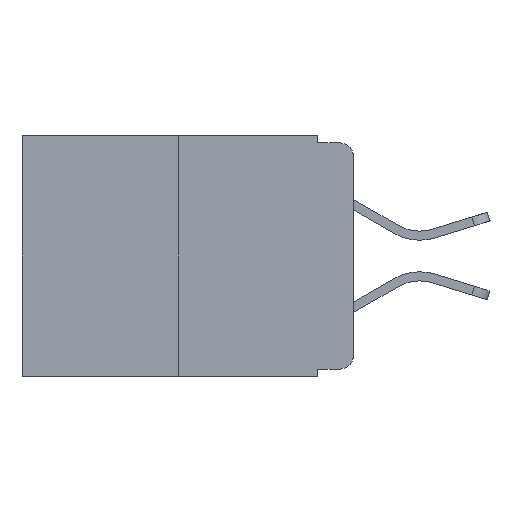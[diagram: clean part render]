
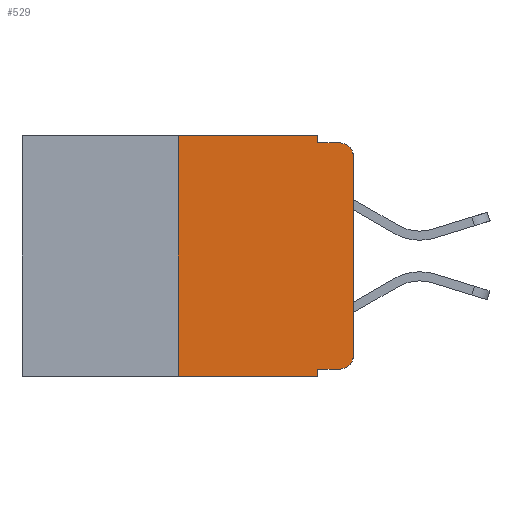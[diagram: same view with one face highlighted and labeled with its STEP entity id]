
A CAD part, left-side view. The second image highlights one B-rep face of the part: STEP entity #529.
In plain terms, the highlighted planar face has unit normal (-1, 0, 0).
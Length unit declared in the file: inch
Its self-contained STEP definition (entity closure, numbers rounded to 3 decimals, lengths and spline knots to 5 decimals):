
#18 = ORIENTED_EDGE ( 'NONE', *, *, #6493, .T. ) ;
#202 = DIRECTION ( 'NONE',  ( 0., 0., 1. ) ) ;
#225 = VERTEX_POINT ( 'NONE', #7910 ) ;
#264 = VERTEX_POINT ( 'NONE', #2748 ) ;
#381 = DIRECTION ( 'NONE',  ( 0., 0., -1. ) ) ;
#408 = VECTOR ( 'NONE', #202, 39.37008 ) ;
#529 = ADVANCED_FACE ( 'NONE', ( #13512 ), #13911, .F. ) ;
#679 = ORIENTED_EDGE ( 'NONE', *, *, #18257, .T. ) ;
#880 = EDGE_CURVE ( 'NONE', #6363, #5729, #3948, .T. ) ;
#1141 = DIRECTION ( 'NONE',  ( 0., 0., -1. ) ) ;
#1307 = VERTEX_POINT ( 'NONE', #15909 ) ;
#1348 = CARTESIAN_POINT ( 'NONE',  ( 0., 0., 0. ) ) ;
#1438 = ORIENTED_EDGE ( 'NONE', *, *, #7384, .F. ) ;
#1807 = VECTOR ( 'NONE', #4282, 39.37008 ) ;
#1952 = CARTESIAN_POINT ( 'NONE',  ( 0., 0.473, -0.343 ) ) ;
#2049 = CARTESIAN_POINT ( 'NONE',  ( 0., 0.25, 0. ) ) ;
#2106 = EDGE_CURVE ( 'NONE', #7403, #9936, #10710, .T. ) ;
#2471 = AXIS2_PLACEMENT_3D ( 'NONE', #18780, #10109, #1141 ) ;
#2748 = CARTESIAN_POINT ( 'NONE',  ( 0., 0.02, -0.01 ) ) ;
#2759 = ORIENTED_EDGE ( 'NONE', *, *, #3079, .T. ) ;
#2834 = CARTESIAN_POINT ( 'NONE',  ( 0., 0.051, 0. ) ) ;
#2950 = CARTESIAN_POINT ( 'NONE',  ( 0., 0.051, 0. ) ) ;
#3002 = EDGE_CURVE ( 'NONE', #5729, #264, #13216, .T. ) ;
#3079 = EDGE_CURVE ( 'NONE', #8422, #1307, #12275, .T. ) ;
#3287 = AXIS2_PLACEMENT_3D ( 'NONE', #10954, #14461, #381 ) ;
#3463 = DIRECTION ( 'NONE',  ( 0., 0., -1. ) ) ;
#3539 = DIRECTION ( 'NONE',  ( 0., 0., 1. ) ) ;
#3898 = ORIENTED_EDGE ( 'NONE', *, *, #2106, .T. ) ;
#3948 = LINE ( 'NONE', #2834, #15300 ) ;
#3957 = VECTOR ( 'NONE', #5284, 39.37008 ) ;
#4106 = ORIENTED_EDGE ( 'NONE', *, *, #3002, .F. ) ;
#4282 = DIRECTION ( 'NONE',  ( 0., -1., 0. ) ) ;
#4502 = DIRECTION ( 'NONE',  ( 0., -1., 0. ) ) ;
#4933 = VERTEX_POINT ( 'NONE', #16500 ) ;
#4966 = DIRECTION ( 'NONE',  ( 0., -1., 0. ) ) ;
#5281 = VECTOR ( 'NONE', #4966, 39.37008 ) ;
#5284 = DIRECTION ( 'NONE',  ( 0., -1., 0. ) ) ;
#5729 = VERTEX_POINT ( 'NONE', #16788 ) ;
#6363 = VERTEX_POINT ( 'NONE', #6462 ) ;
#6462 = CARTESIAN_POINT ( 'NONE',  ( 0., 0.051, 0. ) ) ;
#6493 = EDGE_CURVE ( 'NONE', #225, #4933, #8896, .T. ) ;
#6644 = VECTOR ( 'NONE', #3539, 39.37008 ) ;
#6926 = ORIENTED_EDGE ( 'NONE', *, *, #18538, .F. ) ;
#7085 = DIRECTION ( 'NONE',  ( -1., 0., 0. ) ) ;
#7232 = EDGE_CURVE ( 'NONE', #4933, #8422, #10732, .T. ) ;
#7384 = EDGE_CURVE ( 'NONE', #225, #9936, #15274, .T. ) ;
#7403 = VERTEX_POINT ( 'NONE', #16207 ) ;
#7455 = DIRECTION ( 'NONE',  ( 0., 0., -1. ) ) ;
#7571 = CARTESIAN_POINT ( 'NONE',  ( 0., 0.473, 0. ) ) ;
#7910 = CARTESIAN_POINT ( 'NONE',  ( 0., 0.051, -0.333 ) ) ;
#8422 = VERTEX_POINT ( 'NONE', #15988 ) ;
#8546 = CARTESIAN_POINT ( 'NONE',  ( 0., 0.25, 0. ) ) ;
#8896 = LINE ( 'NONE', #15639, #3957 ) ;
#9852 = AXIS2_PLACEMENT_3D ( 'NONE', #15917, #7085, #17364 ) ;
#9869 = VERTEX_POINT ( 'NONE', #8546 ) ;
#9909 = LINE ( 'NONE', #7571, #13347 ) ;
#9936 = VERTEX_POINT ( 'NONE', #15974 ) ;
#10109 = DIRECTION ( 'NONE',  ( -1., 0., 0. ) ) ;
#10710 = LINE ( 'NONE', #1952, #1807 ) ;
#10732 = CIRCLE ( 'NONE', #2471, 0.02 ) ;
#10757 = EDGE_CURVE ( 'NONE', #9869, #6363, #9909, .T. ) ;
#10954 = CARTESIAN_POINT ( 'NONE',  ( 0., 0.473, 0. ) ) ;
#11420 = VECTOR ( 'NONE', #7455, 39.37008 ) ;
#12275 = LINE ( 'NONE', #1348, #408 ) ;
#12558 = EDGE_LOOP ( 'NONE', ( #2759, #679, #4106, #16148, #14109, #6926, #3898, #1438, #18, #17319 ) ) ;
#13216 = LINE ( 'NONE', #14781, #5281 ) ;
#13347 = VECTOR ( 'NONE', #4502, 39.37008 ) ;
#13512 = FACE_OUTER_BOUND ( 'NONE', #12558, .T. ) ;
#13911 = PLANE ( 'NONE',  #3287 ) ;
#14109 = ORIENTED_EDGE ( 'NONE', *, *, #10757, .F. ) ;
#14461 = DIRECTION ( 'NONE',  ( 1., 0., 0. ) ) ;
#14781 = CARTESIAN_POINT ( 'NONE',  ( 0., 0.051, -0.01 ) ) ;
#15274 = LINE ( 'NONE', #2950, #11420 ) ;
#15300 = VECTOR ( 'NONE', #3463, 39.37008 ) ;
#15639 = CARTESIAN_POINT ( 'NONE',  ( 0., 0.051, -0.333 ) ) ;
#15909 = CARTESIAN_POINT ( 'NONE',  ( 0., 0., -0.03 ) ) ;
#15917 = CARTESIAN_POINT ( 'NONE',  ( 0., 0.02, -0.03 ) ) ;
#15974 = CARTESIAN_POINT ( 'NONE',  ( 0., 0.051, -0.343 ) ) ;
#15988 = CARTESIAN_POINT ( 'NONE',  ( 0., 0., -0.313 ) ) ;
#16117 = CIRCLE ( 'NONE', #9852, 0.02 ) ;
#16148 = ORIENTED_EDGE ( 'NONE', *, *, #880, .F. ) ;
#16207 = CARTESIAN_POINT ( 'NONE',  ( 0., 0.25, -0.343 ) ) ;
#16500 = CARTESIAN_POINT ( 'NONE',  ( 0., 0.02, -0.333 ) ) ;
#16788 = CARTESIAN_POINT ( 'NONE',  ( 0., 0.051, -0.01 ) ) ;
#17319 = ORIENTED_EDGE ( 'NONE', *, *, #7232, .T. ) ;
#17364 = DIRECTION ( 'NONE',  ( 0., 0., -1. ) ) ;
#18257 = EDGE_CURVE ( 'NONE', #1307, #264, #16117, .T. ) ;
#18350 = LINE ( 'NONE', #2049, #6644 ) ;
#18538 = EDGE_CURVE ( 'NONE', #7403, #9869, #18350, .T. ) ;
#18780 = CARTESIAN_POINT ( 'NONE',  ( 0., 0.02, -0.313 ) ) ;
